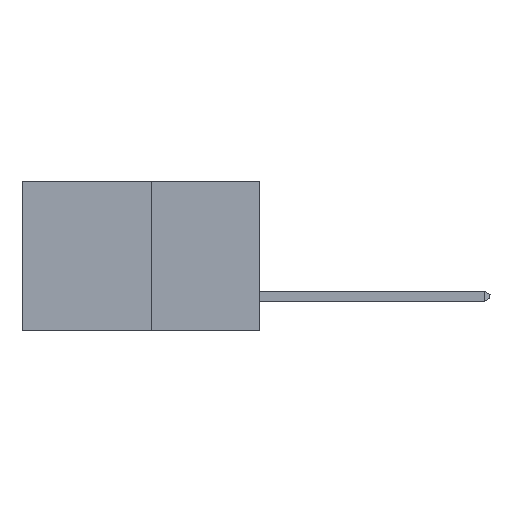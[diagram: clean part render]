
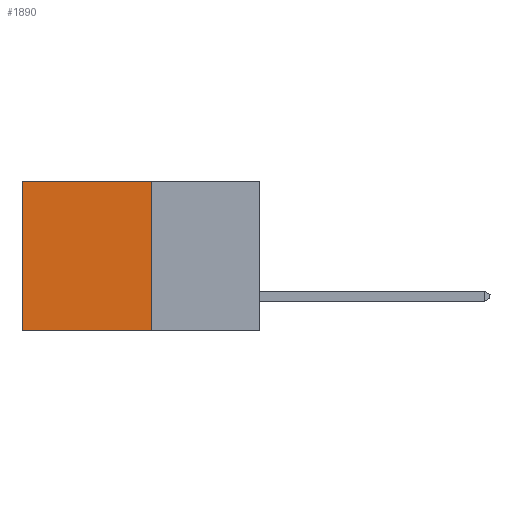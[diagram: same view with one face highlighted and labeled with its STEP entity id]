
A CAD part, left-side view. The second image highlights one B-rep face of the part: STEP entity #1890.
In plain terms, the highlighted planar face has unit normal (-1, 0, 0).
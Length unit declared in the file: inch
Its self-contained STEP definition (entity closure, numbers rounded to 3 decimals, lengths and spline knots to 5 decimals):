
#164 = EDGE_CURVE ( 'NONE', #10243, #8853, #8773, .T. ) ;
#461 = CARTESIAN_POINT ( 'NONE',  ( 0.277, 0.27, -0.37 ) ) ;
#529 = DIRECTION ( 'NONE',  ( 0., 0., -1. ) ) ;
#578 = LINE ( 'NONE', #9697, #5640 ) ;
#675 = ORIENTED_EDGE ( 'NONE', *, *, #8811, .F. ) ;
#1017 = LINE ( 'NONE', #8146, #10675 ) ;
#1890 = ADVANCED_FACE ( 'NONE', ( #8306 ), #1930, .F. ) ;
#1930 = PLANE ( 'NONE',  #6591 ) ;
#2177 = EDGE_LOOP ( 'NONE', ( #11377, #8935, #675, #8697 ) ) ;
#3426 = DIRECTION ( 'NONE',  ( 0., 0., -1. ) ) ;
#4476 = EDGE_CURVE ( 'NONE', #10116, #10243, #578, .T. ) ;
#4821 = VERTEX_POINT ( 'NONE', #7082 ) ;
#4972 = LINE ( 'NONE', #7601, #7824 ) ;
#5374 = CARTESIAN_POINT ( 'NONE',  ( 0.277, 0.59, -0.37 ) ) ;
#5394 = CARTESIAN_POINT ( 'NONE',  ( 0.277, 0.59, -0.37 ) ) ;
#5640 = VECTOR ( 'NONE', #9612, 39.37008 ) ;
#5647 = DIRECTION ( 'NONE',  ( 1., 0., 0. ) ) ;
#6591 = AXIS2_PLACEMENT_3D ( 'NONE', #461, #5647, #529 ) ;
#6947 = EDGE_CURVE ( 'NONE', #4821, #8853, #4972, .T. ) ;
#7082 = CARTESIAN_POINT ( 'NONE',  ( 0.277, 0.27, -0.37 ) ) ;
#7561 = DIRECTION ( 'NONE',  ( 0., 1., 0. ) ) ;
#7601 = CARTESIAN_POINT ( 'NONE',  ( 0.277, 0.27, -0.37 ) ) ;
#7660 = DIRECTION ( 'NONE',  ( 0., 0., -1. ) ) ;
#7824 = VECTOR ( 'NONE', #7561, 39.37008 ) ;
#8146 = CARTESIAN_POINT ( 'NONE',  ( 0.277, 0.27, -0.37 ) ) ;
#8306 = FACE_OUTER_BOUND ( 'NONE', #2177, .T. ) ;
#8480 = VECTOR ( 'NONE', #7660, 39.37008 ) ;
#8697 = ORIENTED_EDGE ( 'NONE', *, *, #4476, .T. ) ;
#8773 = LINE ( 'NONE', #5394, #8480 ) ;
#8811 = EDGE_CURVE ( 'NONE', #10116, #4821, #1017, .T. ) ;
#8853 = VERTEX_POINT ( 'NONE', #5374 ) ;
#8935 = ORIENTED_EDGE ( 'NONE', *, *, #6947, .F. ) ;
#9612 = DIRECTION ( 'NONE',  ( 0., 1., 0. ) ) ;
#9697 = CARTESIAN_POINT ( 'NONE',  ( 0.277, 0.27, 0. ) ) ;
#10116 = VERTEX_POINT ( 'NONE', #12245 ) ;
#10243 = VERTEX_POINT ( 'NONE', #10687 ) ;
#10675 = VECTOR ( 'NONE', #3426, 39.37008 ) ;
#10687 = CARTESIAN_POINT ( 'NONE',  ( 0.277, 0.59, 0. ) ) ;
#11377 = ORIENTED_EDGE ( 'NONE', *, *, #164, .T. ) ;
#12245 = CARTESIAN_POINT ( 'NONE',  ( 0.277, 0.27, 0. ) ) ;
